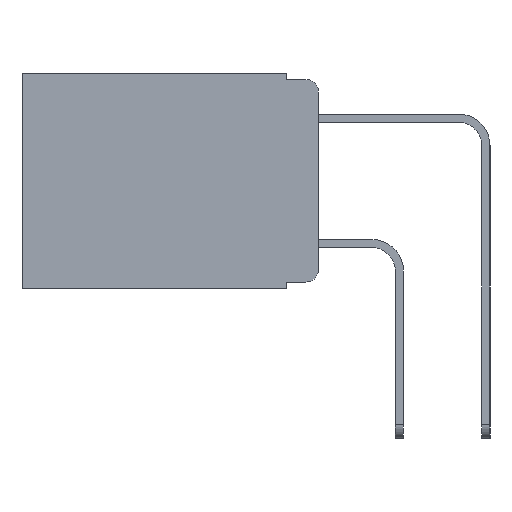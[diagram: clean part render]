
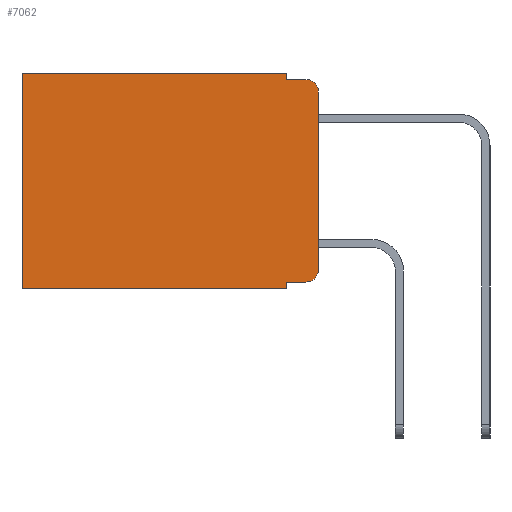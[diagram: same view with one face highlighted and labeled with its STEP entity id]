
A CAD part, left-side view. The second image highlights one B-rep face of the part: STEP entity #7062.
In plain terms, the highlighted planar face has unit normal (-1, 0, 0).
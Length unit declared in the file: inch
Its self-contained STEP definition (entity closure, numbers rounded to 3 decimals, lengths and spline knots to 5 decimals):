
#138 = VERTEX_POINT ( 'NONE', #1067 ) ;
#242 = ORIENTED_EDGE ( 'NONE', *, *, #18666, .T. ) ;
#300 = DIRECTION ( 'NONE',  ( -1., 0., 0. ) ) ;
#446 = ORIENTED_EDGE ( 'NONE', *, *, #12645, .T. ) ;
#710 = DIRECTION ( 'NONE',  ( 0., 0., -1. ) ) ;
#958 = DIRECTION ( 'NONE',  ( 0., -1., 0. ) ) ;
#974 = CARTESIAN_POINT ( 'NONE',  ( 0.298, 0.02, -0.03 ) ) ;
#1067 = CARTESIAN_POINT ( 'NONE',  ( 0.298, 0.02, -0.01 ) ) ;
#1192 = ORIENTED_EDGE ( 'NONE', *, *, #13727, .F. ) ;
#1425 = VERTEX_POINT ( 'NONE', #13834 ) ;
#2199 = DIRECTION ( 'NONE',  ( 0., 1., 0. ) ) ;
#2317 = VERTEX_POINT ( 'NONE', #2411 ) ;
#2334 = DIRECTION ( 'NONE',  ( 0., 1., 0. ) ) ;
#2411 = CARTESIAN_POINT ( 'NONE',  ( 0.298, 0.051, -0.01 ) ) ;
#2676 = DIRECTION ( 'NONE',  ( 0., 0., -1. ) ) ;
#2820 = DIRECTION ( 'NONE',  ( 0., 0., -1. ) ) ;
#3762 = CARTESIAN_POINT ( 'NONE',  ( 0.298, 0., 0. ) ) ;
#4296 = CARTESIAN_POINT ( 'NONE',  ( 0.298, 0.051, -0.01 ) ) ;
#4784 = VECTOR ( 'NONE', #5353, 39.37008 ) ;
#4856 = EDGE_CURVE ( 'NONE', #6755, #6214, #4861, .T. ) ;
#4861 = LINE ( 'NONE', #17237, #8991 ) ;
#5097 = CARTESIAN_POINT ( 'NONE',  ( 0.298, 0.473, 0. ) ) ;
#5353 = DIRECTION ( 'NONE',  ( 0., 0., -1. ) ) ;
#6106 = LINE ( 'NONE', #13475, #17454 ) ;
#6214 = VERTEX_POINT ( 'NONE', #7975 ) ;
#6755 = VERTEX_POINT ( 'NONE', #9172 ) ;
#7062 = ADVANCED_FACE ( 'NONE', ( #9361 ), #14570, .F. ) ;
#7091 = AXIS2_PLACEMENT_3D ( 'NONE', #7160, #10193, #710 ) ;
#7160 = CARTESIAN_POINT ( 'NONE',  ( 0.298, 0., 0. ) ) ;
#7896 = EDGE_CURVE ( 'NONE', #8799, #6214, #17981, .T. ) ;
#7975 = CARTESIAN_POINT ( 'NONE',  ( 0.298, 0.473, -0.343 ) ) ;
#8073 = VECTOR ( 'NONE', #2334, 39.37008 ) ;
#8799 = VERTEX_POINT ( 'NONE', #5097 ) ;
#8836 = ORIENTED_EDGE ( 'NONE', *, *, #15542, .T. ) ;
#8991 = VECTOR ( 'NONE', #2199, 39.37008 ) ;
#9172 = CARTESIAN_POINT ( 'NONE',  ( 0.298, 0.051, -0.343 ) ) ;
#9360 = VERTEX_POINT ( 'NONE', #13079 ) ;
#9361 = FACE_OUTER_BOUND ( 'NONE', #17412, .T. ) ;
#9475 = LINE ( 'NONE', #4296, #12936 ) ;
#9646 = AXIS2_PLACEMENT_3D ( 'NONE', #9873, #300, #11329 ) ;
#9663 = ORIENTED_EDGE ( 'NONE', *, *, #19408, .F. ) ;
#9873 = CARTESIAN_POINT ( 'NONE',  ( 0.298, 0.02, -0.313 ) ) ;
#10105 = CARTESIAN_POINT ( 'NONE',  ( 0.298, 0., 0. ) ) ;
#10188 = VERTEX_POINT ( 'NONE', #10586 ) ;
#10193 = DIRECTION ( 'NONE',  ( 1., 0., 0. ) ) ;
#10318 = ORIENTED_EDGE ( 'NONE', *, *, #4856, .F. ) ;
#10586 = CARTESIAN_POINT ( 'NONE',  ( 0.298, 0., -0.03 ) ) ;
#10654 = ORIENTED_EDGE ( 'NONE', *, *, #7896, .T. ) ;
#11329 = DIRECTION ( 'NONE',  ( 0., 0., -1. ) ) ;
#11869 = DIRECTION ( 'NONE',  ( -1., 0., 0. ) ) ;
#12286 = ORIENTED_EDGE ( 'NONE', *, *, #17739, .F. ) ;
#12492 = CIRCLE ( 'NONE', #9646, 0.02 ) ;
#12496 = LINE ( 'NONE', #10105, #8073 ) ;
#12645 = EDGE_CURVE ( 'NONE', #10188, #138, #14020, .T. ) ;
#12936 = VECTOR ( 'NONE', #958, 39.37008 ) ;
#12957 = VECTOR ( 'NONE', #18778, 39.37008 ) ;
#13079 = CARTESIAN_POINT ( 'NONE',  ( 0.298, 0.051, -0.333 ) ) ;
#13475 = CARTESIAN_POINT ( 'NONE',  ( 0.298, 0.051, 0. ) ) ;
#13544 = CARTESIAN_POINT ( 'NONE',  ( 0.298, 0.051, 0. ) ) ;
#13692 = VECTOR ( 'NONE', #2820, 39.37008 ) ;
#13727 = EDGE_CURVE ( 'NONE', #10188, #1425, #16698, .T. ) ;
#13834 = CARTESIAN_POINT ( 'NONE',  ( 0.298, 0., -0.313 ) ) ;
#14020 = CIRCLE ( 'NONE', #18836, 0.02 ) ;
#14065 = VERTEX_POINT ( 'NONE', #17986 ) ;
#14072 = ORIENTED_EDGE ( 'NONE', *, *, #18067, .T. ) ;
#14570 = PLANE ( 'NONE',  #7091 ) ;
#14958 = DIRECTION ( 'NONE',  ( 0., 0., -1. ) ) ;
#15075 = VECTOR ( 'NONE', #17848, 39.37008 ) ;
#15526 = LINE ( 'NONE', #16412, #15075 ) ;
#15542 = EDGE_CURVE ( 'NONE', #9360, #14065, #15526, .T. ) ;
#16412 = CARTESIAN_POINT ( 'NONE',  ( 0.298, 0.051, -0.333 ) ) ;
#16432 = CARTESIAN_POINT ( 'NONE',  ( 0.298, 0.473, 0. ) ) ;
#16698 = LINE ( 'NONE', #3762, #4784 ) ;
#17142 = EDGE_CURVE ( 'NONE', #19504, #2317, #17262, .T. ) ;
#17237 = CARTESIAN_POINT ( 'NONE',  ( 0.298, 0., -0.343 ) ) ;
#17262 = LINE ( 'NONE', #17344, #12957 ) ;
#17344 = CARTESIAN_POINT ( 'NONE',  ( 0.298, 0.051, 0. ) ) ;
#17412 = EDGE_LOOP ( 'NONE', ( #1192, #446, #9663, #18232, #242, #10654, #10318, #12286, #8836, #14072 ) ) ;
#17454 = VECTOR ( 'NONE', #14958, 39.37008 ) ;
#17739 = EDGE_CURVE ( 'NONE', #9360, #6755, #6106, .T. ) ;
#17848 = DIRECTION ( 'NONE',  ( 0., -1., 0. ) ) ;
#17981 = LINE ( 'NONE', #16432, #13692 ) ;
#17986 = CARTESIAN_POINT ( 'NONE',  ( 0.298, 0.02, -0.333 ) ) ;
#18067 = EDGE_CURVE ( 'NONE', #14065, #1425, #12492, .T. ) ;
#18232 = ORIENTED_EDGE ( 'NONE', *, *, #17142, .F. ) ;
#18666 = EDGE_CURVE ( 'NONE', #19504, #8799, #12496, .T. ) ;
#18778 = DIRECTION ( 'NONE',  ( 0., 0., -1. ) ) ;
#18836 = AXIS2_PLACEMENT_3D ( 'NONE', #974, #11869, #2676 ) ;
#19408 = EDGE_CURVE ( 'NONE', #2317, #138, #9475, .T. ) ;
#19504 = VERTEX_POINT ( 'NONE', #13544 ) ;
